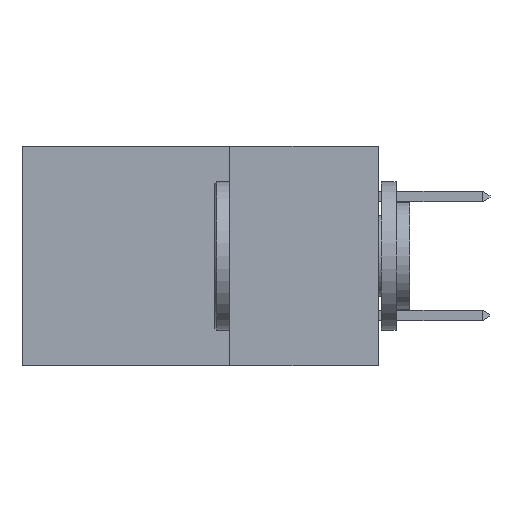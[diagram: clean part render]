
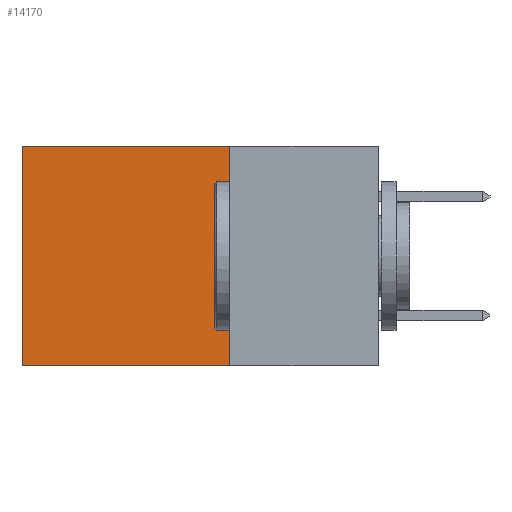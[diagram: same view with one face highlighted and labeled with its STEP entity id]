
A CAD part, left-side view. The second image highlights one B-rep face of the part: STEP entity #14170.
In plain terms, the highlighted planar face has unit normal (-1, 0, 0).
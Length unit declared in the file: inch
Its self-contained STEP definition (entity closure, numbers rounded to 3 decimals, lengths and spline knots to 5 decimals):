
#154 = EDGE_LOOP ( 'NONE', ( #1750, #18640, #5719, #18524 ) ) ;
#1750 = ORIENTED_EDGE ( 'NONE', *, *, #9240, .T. ) ;
#2350 = VECTOR ( 'NONE', #6569, 39.37008 ) ;
#3913 = VECTOR ( 'NONE', #18729, 39.37008 ) ;
#5206 = DIRECTION ( 'NONE',  ( 0., 1., 0. ) ) ;
#5364 = EDGE_CURVE ( 'NONE', #15634, #10077, #15712, .T. ) ;
#5719 = ORIENTED_EDGE ( 'NONE', *, *, #10224, .F. ) ;
#5988 = PLANE ( 'NONE',  #17320 ) ;
#6247 = EDGE_CURVE ( 'NONE', #15581, #7286, #7050, .T. ) ;
#6569 = DIRECTION ( 'NONE',  ( 0., 1., 0. ) ) ;
#6618 = VECTOR ( 'NONE', #17918, 39.37008 ) ;
#7050 = LINE ( 'NONE', #16497, #15671 ) ;
#7286 = VERTEX_POINT ( 'NONE', #17526 ) ;
#7570 = DIRECTION ( 'NONE',  ( 1., 0., 0. ) ) ;
#7699 = FACE_OUTER_BOUND ( 'NONE', #154, .T. ) ;
#8306 = CARTESIAN_POINT ( 'NONE',  ( 0.298, 0.25, 0. ) ) ;
#9240 = EDGE_CURVE ( 'NONE', #10077, #7286, #20213, .T. ) ;
#10077 = VERTEX_POINT ( 'NONE', #11225 ) ;
#10224 = EDGE_CURVE ( 'NONE', #15634, #15581, #11371, .T. ) ;
#11225 = CARTESIAN_POINT ( 'NONE',  ( 0.298, 0.6, 0. ) ) ;
#11371 = LINE ( 'NONE', #8306, #6618 ) ;
#11697 = CARTESIAN_POINT ( 'NONE',  ( 0.298, 0.25, 0. ) ) ;
#12431 = CARTESIAN_POINT ( 'NONE',  ( 0.298, 0.6, 0. ) ) ;
#13190 = CARTESIAN_POINT ( 'NONE',  ( 0.298, 0.25, -0.37 ) ) ;
#14170 = ADVANCED_FACE ( 'NONE', ( #7699 ), #5988, .F. ) ;
#15581 = VERTEX_POINT ( 'NONE', #13190 ) ;
#15634 = VERTEX_POINT ( 'NONE', #11697 ) ;
#15671 = VECTOR ( 'NONE', #5206, 39.37008 ) ;
#15712 = LINE ( 'NONE', #16263, #2350 ) ;
#16263 = CARTESIAN_POINT ( 'NONE',  ( 0.298, 0.25, 0. ) ) ;
#16497 = CARTESIAN_POINT ( 'NONE',  ( 0.298, 0.25, -0.37 ) ) ;
#17239 = CARTESIAN_POINT ( 'NONE',  ( 0.298, 0.25, 0. ) ) ;
#17320 = AXIS2_PLACEMENT_3D ( 'NONE', #17239, #7570, #18706 ) ;
#17526 = CARTESIAN_POINT ( 'NONE',  ( 0.298, 0.6, -0.37 ) ) ;
#17918 = DIRECTION ( 'NONE',  ( 0., 0., -1. ) ) ;
#18524 = ORIENTED_EDGE ( 'NONE', *, *, #5364, .T. ) ;
#18640 = ORIENTED_EDGE ( 'NONE', *, *, #6247, .F. ) ;
#18706 = DIRECTION ( 'NONE',  ( 0., 0., -1. ) ) ;
#18729 = DIRECTION ( 'NONE',  ( 0., 0., -1. ) ) ;
#20213 = LINE ( 'NONE', #12431, #3913 ) ;
